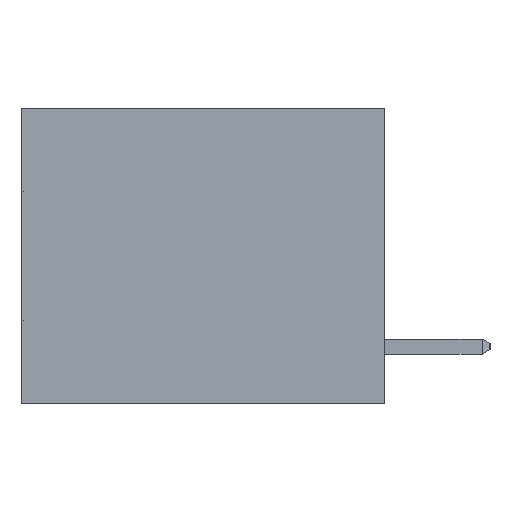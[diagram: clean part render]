
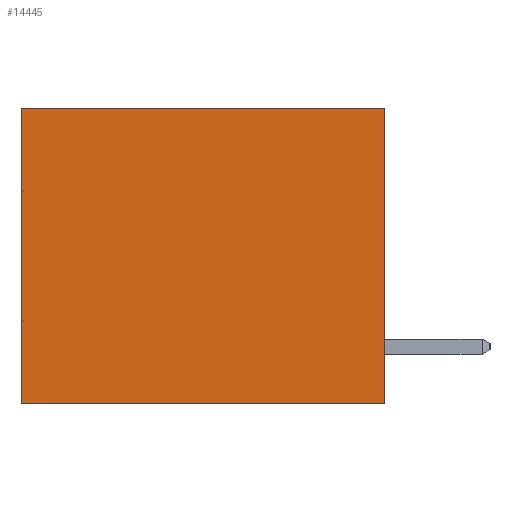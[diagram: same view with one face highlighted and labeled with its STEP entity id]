
A CAD part, left-side view. The second image highlights one B-rep face of the part: STEP entity #14445.
In plain terms, the highlighted planar face has unit normal (-1, 0, 0).
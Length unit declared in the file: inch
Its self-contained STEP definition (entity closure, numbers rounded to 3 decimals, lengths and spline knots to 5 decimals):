
#64 = CARTESIAN_POINT ( 'NONE',  ( 0.3165, 0., -0.49 ) ) ;
#445 = LINE ( 'NONE', #28711, #827 ) ;
#827 = VECTOR ( 'NONE', #24187, 39.37008 ) ;
#1369 = VERTEX_POINT ( 'NONE', #18792 ) ;
#2016 = EDGE_CURVE ( 'NONE', #27965, #16216, #445, .T. ) ;
#4098 = LINE ( 'NONE', #27029, #22013 ) ;
#4667 = EDGE_CURVE ( 'NONE', #1369, #13643, #4098, .T. ) ;
#4675 = FACE_OUTER_BOUND ( 'NONE', #29338, .T. ) ;
#5508 = ORIENTED_EDGE ( 'NONE', *, *, #9896, .F. ) ;
#6056 = EDGE_CURVE ( 'NONE', #1369, #27965, #14147, .T. ) ;
#8526 = CARTESIAN_POINT ( 'NONE',  ( 0.3165, 0., -0.49 ) ) ;
#8892 = CARTESIAN_POINT ( 'NONE',  ( 0.3165, 0., -0.49 ) ) ;
#9643 = LINE ( 'NONE', #8892, #21872 ) ;
#9896 = EDGE_CURVE ( 'NONE', #13643, #16216, #9643, .T. ) ;
#10488 = ORIENTED_EDGE ( 'NONE', *, *, #6056, .T. ) ;
#12370 = CARTESIAN_POINT ( 'NONE',  ( 0.3165, 0.6, -0.49 ) ) ;
#13643 = VERTEX_POINT ( 'NONE', #64 ) ;
#13869 = CARTESIAN_POINT ( 'NONE',  ( 0.3165, 0., 0. ) ) ;
#14147 = LINE ( 'NONE', #13869, #21370 ) ;
#14279 = DIRECTION ( 'NONE',  ( 0., 1., 0. ) ) ;
#14445 = ADVANCED_FACE ( 'NONE', ( #4675 ), #26048, .F. ) ;
#15835 = CARTESIAN_POINT ( 'NONE',  ( 0.3165, 0.6, 0. ) ) ;
#16216 = VERTEX_POINT ( 'NONE', #12370 ) ;
#18792 = CARTESIAN_POINT ( 'NONE',  ( 0.3165, 0., 0. ) ) ;
#19745 = DIRECTION ( 'NONE',  ( 0., 0., -1. ) ) ;
#21370 = VECTOR ( 'NONE', #14279, 39.37008 ) ;
#21872 = VECTOR ( 'NONE', #23413, 39.37008 ) ;
#22013 = VECTOR ( 'NONE', #19745, 39.37008 ) ;
#23413 = DIRECTION ( 'NONE',  ( 0., 1., 0. ) ) ;
#24187 = DIRECTION ( 'NONE',  ( 0., 0., -1. ) ) ;
#25716 = AXIS2_PLACEMENT_3D ( 'NONE', #8526, #30539, #28303 ) ;
#26048 = PLANE ( 'NONE',  #25716 ) ;
#27029 = CARTESIAN_POINT ( 'NONE',  ( 0.3165, 0., -0.49 ) ) ;
#27965 = VERTEX_POINT ( 'NONE', #15835 ) ;
#28303 = DIRECTION ( 'NONE',  ( 0., 0., -1. ) ) ;
#28711 = CARTESIAN_POINT ( 'NONE',  ( 0.3165, 0.6, -0.49 ) ) ;
#29307 = ORIENTED_EDGE ( 'NONE', *, *, #4667, .F. ) ;
#29338 = EDGE_LOOP ( 'NONE', ( #30963, #5508, #29307, #10488 ) ) ;
#30539 = DIRECTION ( 'NONE',  ( 1., 0., 0. ) ) ;
#30963 = ORIENTED_EDGE ( 'NONE', *, *, #2016, .T. ) ;
